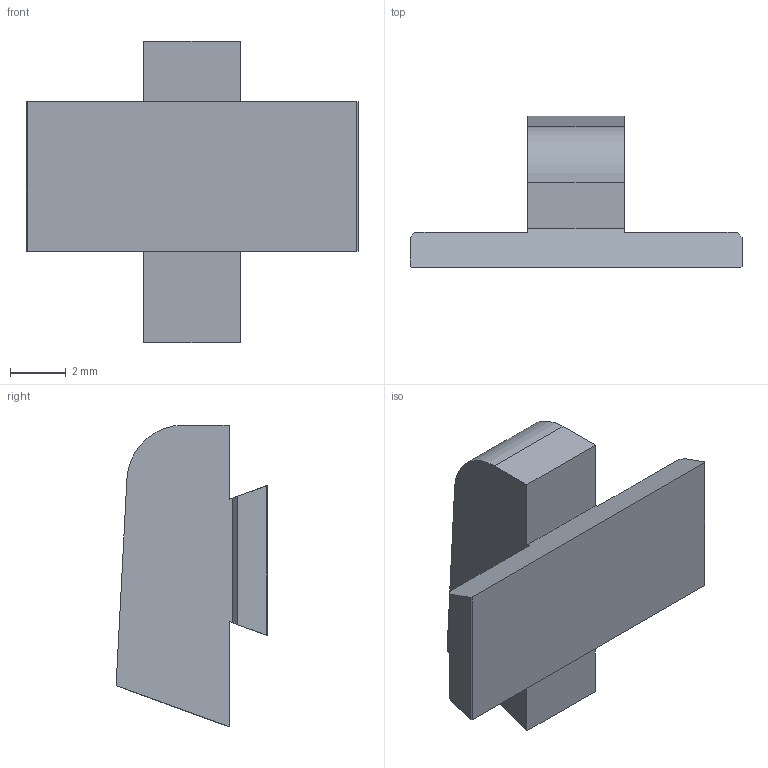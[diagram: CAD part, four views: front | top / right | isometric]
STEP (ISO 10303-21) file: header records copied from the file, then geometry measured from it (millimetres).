
FILE_DESCRIPTION (( 'STEP AP214' ), '1' );
FILE_NAME ('SIGHTS - TRIJICON FRONT.STEP', '2013-06-19T14:00:34', ( 'Asher' ), ( '' ), 'SwSTEP 2.0', 'SolidWorks 2013', '' );
FILE_SCHEMA (( 'AUTOMOTIVE_DESIGN' ));
Length unit declared in the file: millimetre
Products named in the file (1): SIGHTS - TRIJICON FRONT
Bounding box: 11.94 x 5.46 x 10.85 mm (x, y, z)
Volume: 201.2 mm3; surface area: 322.4 mm2
Topology: 1 solids, 1 shells, 25 faces, 63 edges, 42 vertices
Faces by surface type: plane 20, cylinder 5
Entity records: 779 total; most frequent: CARTESIAN_POINT 137, ORIENTED_EDGE 126, DIRECTION 121, EDGE_CURVE 63, VECTOR 53, LINE 53, VERTEX_POINT 42, AXIS2_PLACEMENT_3D 34
